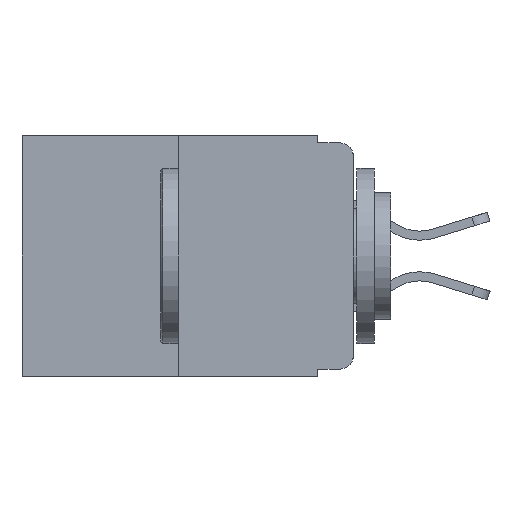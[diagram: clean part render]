
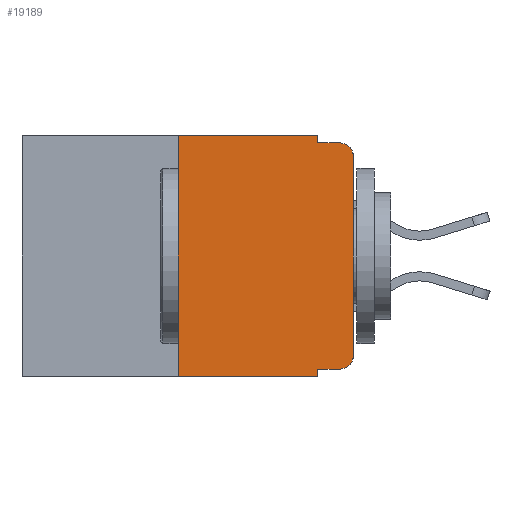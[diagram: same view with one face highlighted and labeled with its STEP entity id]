
A CAD part, left-side view. The second image highlights one B-rep face of the part: STEP entity #19189.
In plain terms, the highlighted planar face has unit normal (-1, 0, 0).
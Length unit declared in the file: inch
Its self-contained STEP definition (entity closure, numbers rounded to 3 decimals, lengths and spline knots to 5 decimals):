
#102 = EDGE_CURVE ( 'NONE', #18604, #19914, #8652, .T. ) ;
#125 = CARTESIAN_POINT ( 'NONE',  ( 0., 0.051, 0. ) ) ;
#258 = DIRECTION ( 'NONE',  ( 0., 0., -1. ) ) ;
#691 = DIRECTION ( 'NONE',  ( 0., 0., -1. ) ) ;
#784 = EDGE_CURVE ( 'NONE', #911, #15197, #15744, .T. ) ;
#889 = VERTEX_POINT ( 'NONE', #9720 ) ;
#911 = VERTEX_POINT ( 'NONE', #6994 ) ;
#1133 = DIRECTION ( 'NONE',  ( 0., -1., 0. ) ) ;
#1774 = CARTESIAN_POINT ( 'NONE',  ( 0., 0., -0.03 ) ) ;
#1929 = PLANE ( 'NONE',  #3687 ) ;
#2467 = DIRECTION ( 'NONE',  ( 0., 0., -1. ) ) ;
#2646 = ORIENTED_EDGE ( 'NONE', *, *, #784, .F. ) ;
#2663 = DIRECTION ( 'NONE',  ( 0., -1., 0. ) ) ;
#2829 = ORIENTED_EDGE ( 'NONE', *, *, #102, .T. ) ;
#3432 = DIRECTION ( 'NONE',  ( 0., -1., 0. ) ) ;
#3687 = AXIS2_PLACEMENT_3D ( 'NONE', #9559, #14541, #691 ) ;
#3774 = VERTEX_POINT ( 'NONE', #4260 ) ;
#4103 = DIRECTION ( 'NONE',  ( 0., -1., 0. ) ) ;
#4203 = LINE ( 'NONE', #13228, #6293 ) ;
#4260 = CARTESIAN_POINT ( 'NONE',  ( 0., 0.02, -0.01 ) ) ;
#4546 = EDGE_LOOP ( 'NONE', ( #16401, #16192, #6330, #9110, #2646, #13337, #2829, #17580, #14729, #10602 ) ) ;
#5064 = EDGE_CURVE ( 'NONE', #9817, #7848, #13394, .T. ) ;
#5189 = FACE_OUTER_BOUND ( 'NONE', #4546, .T. ) ;
#5724 = VECTOR ( 'NONE', #3432, 39.37008 ) ;
#5832 = LINE ( 'NONE', #8758, #7526 ) ;
#5865 = DIRECTION ( 'NONE',  ( 0., 0., 1. ) ) ;
#6293 = VECTOR ( 'NONE', #2663, 39.37008 ) ;
#6330 = ORIENTED_EDGE ( 'NONE', *, *, #18924, .F. ) ;
#6994 = CARTESIAN_POINT ( 'NONE',  ( 0., 0.25, 0. ) ) ;
#7526 = VECTOR ( 'NONE', #4103, 39.37008 ) ;
#7833 = LINE ( 'NONE', #17516, #13676 ) ;
#7848 = VERTEX_POINT ( 'NONE', #1774 ) ;
#7899 = AXIS2_PLACEMENT_3D ( 'NONE', #19581, #10191, #2467 ) ;
#8221 = VECTOR ( 'NONE', #1133, 39.37008 ) ;
#8652 = LINE ( 'NONE', #14870, #8221 ) ;
#8758 = CARTESIAN_POINT ( 'NONE',  ( 0., 0.051, -0.333 ) ) ;
#9110 = ORIENTED_EDGE ( 'NONE', *, *, #12360, .F. ) ;
#9153 = CARTESIAN_POINT ( 'NONE',  ( 0., 0., -0.313 ) ) ;
#9425 = EDGE_CURVE ( 'NONE', #7848, #3774, #15930, .T. ) ;
#9559 = CARTESIAN_POINT ( 'NONE',  ( 0., 0.473, 0. ) ) ;
#9585 = CARTESIAN_POINT ( 'NONE',  ( 0., 0.25, -0.343 ) ) ;
#9621 = VECTOR ( 'NONE', #19960, 39.37008 ) ;
#9715 = LINE ( 'NONE', #13884, #16061 ) ;
#9720 = CARTESIAN_POINT ( 'NONE',  ( 0., 0.02, -0.333 ) ) ;
#9817 = VERTEX_POINT ( 'NONE', #9153 ) ;
#10191 = DIRECTION ( 'NONE',  ( -1., 0., 0. ) ) ;
#10536 = CARTESIAN_POINT ( 'NONE',  ( 0., 0.02, -0.03 ) ) ;
#10602 = ORIENTED_EDGE ( 'NONE', *, *, #18954, .T. ) ;
#11742 = CARTESIAN_POINT ( 'NONE',  ( 0., 0.25, 0. ) ) ;
#12142 = VERTEX_POINT ( 'NONE', #13159 ) ;
#12251 = CARTESIAN_POINT ( 'NONE',  ( 0., 0.051, -0.343 ) ) ;
#12360 = EDGE_CURVE ( 'NONE', #15197, #14081, #7833, .T. ) ;
#12510 = DIRECTION ( 'NONE',  ( 0., 0., -1. ) ) ;
#12572 = CARTESIAN_POINT ( 'NONE',  ( 0., 0.473, 0. ) ) ;
#12651 = AXIS2_PLACEMENT_3D ( 'NONE', #10536, #15414, #15218 ) ;
#13159 = CARTESIAN_POINT ( 'NONE',  ( 0., 0.051, -0.333 ) ) ;
#13228 = CARTESIAN_POINT ( 'NONE',  ( 0., 0.051, -0.01 ) ) ;
#13337 = ORIENTED_EDGE ( 'NONE', *, *, #13651, .F. ) ;
#13394 = LINE ( 'NONE', #13689, #9621 ) ;
#13651 = EDGE_CURVE ( 'NONE', #18604, #911, #17989, .T. ) ;
#13676 = VECTOR ( 'NONE', #12510, 39.37008 ) ;
#13689 = CARTESIAN_POINT ( 'NONE',  ( 0., 0., 0. ) ) ;
#13707 = VECTOR ( 'NONE', #5865, 39.37008 ) ;
#13884 = CARTESIAN_POINT ( 'NONE',  ( 0., 0.051, 0. ) ) ;
#14081 = VERTEX_POINT ( 'NONE', #14887 ) ;
#14541 = DIRECTION ( 'NONE',  ( 1., 0., 0. ) ) ;
#14725 = EDGE_CURVE ( 'NONE', #12142, #19914, #9715, .T. ) ;
#14729 = ORIENTED_EDGE ( 'NONE', *, *, #17554, .T. ) ;
#14870 = CARTESIAN_POINT ( 'NONE',  ( 0., 0.473, -0.343 ) ) ;
#14887 = CARTESIAN_POINT ( 'NONE',  ( 0., 0.051, -0.01 ) ) ;
#15197 = VERTEX_POINT ( 'NONE', #125 ) ;
#15218 = DIRECTION ( 'NONE',  ( 0., 0., -1. ) ) ;
#15414 = DIRECTION ( 'NONE',  ( -1., 0., 0. ) ) ;
#15744 = LINE ( 'NONE', #12572, #5724 ) ;
#15930 = CIRCLE ( 'NONE', #12651, 0.02 ) ;
#16061 = VECTOR ( 'NONE', #258, 39.37008 ) ;
#16192 = ORIENTED_EDGE ( 'NONE', *, *, #9425, .T. ) ;
#16401 = ORIENTED_EDGE ( 'NONE', *, *, #5064, .T. ) ;
#17516 = CARTESIAN_POINT ( 'NONE',  ( 0., 0.051, 0. ) ) ;
#17554 = EDGE_CURVE ( 'NONE', #12142, #889, #5832, .T. ) ;
#17580 = ORIENTED_EDGE ( 'NONE', *, *, #14725, .F. ) ;
#17684 = CIRCLE ( 'NONE', #7899, 0.02 ) ;
#17989 = LINE ( 'NONE', #11742, #13707 ) ;
#18604 = VERTEX_POINT ( 'NONE', #9585 ) ;
#18924 = EDGE_CURVE ( 'NONE', #14081, #3774, #4203, .T. ) ;
#18954 = EDGE_CURVE ( 'NONE', #889, #9817, #17684, .T. ) ;
#19189 = ADVANCED_FACE ( 'NONE', ( #5189 ), #1929, .F. ) ;
#19581 = CARTESIAN_POINT ( 'NONE',  ( 0., 0.02, -0.313 ) ) ;
#19914 = VERTEX_POINT ( 'NONE', #12251 ) ;
#19960 = DIRECTION ( 'NONE',  ( 0., 0., 1. ) ) ;
